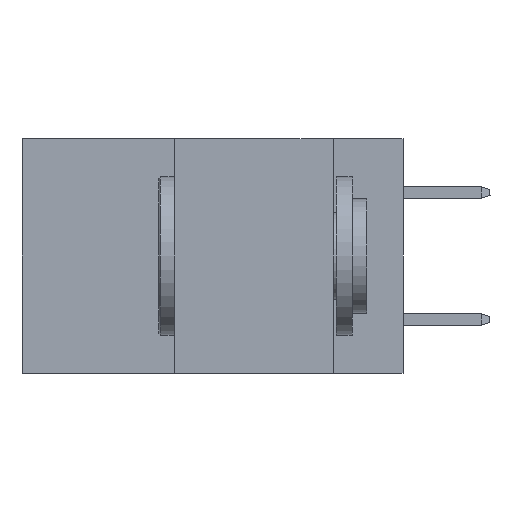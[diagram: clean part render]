
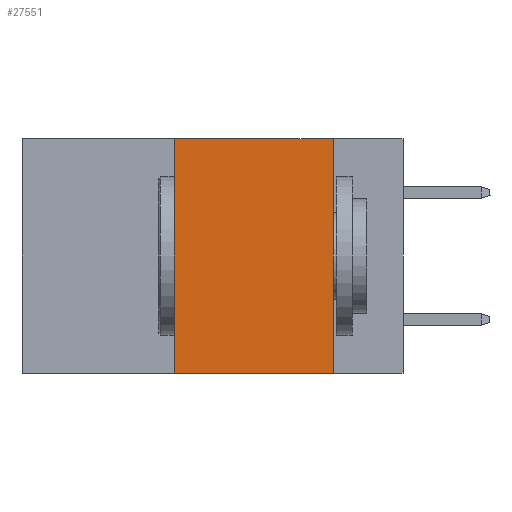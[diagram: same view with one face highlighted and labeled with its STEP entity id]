
A CAD part, left-side view. The second image highlights one B-rep face of the part: STEP entity #27551.
In plain terms, the highlighted planar face has unit normal (-1, 0, 0).
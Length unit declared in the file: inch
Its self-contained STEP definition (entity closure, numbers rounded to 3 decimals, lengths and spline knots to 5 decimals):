
#116 = AXIS2_PLACEMENT_3D ( 'NONE', #1748, #18415, #23609 ) ;
#1748 = CARTESIAN_POINT ( 'NONE',  ( 0., 0.6, 0. ) ) ;
#1804 = DIRECTION ( 'NONE',  ( 0., 0., -1. ) ) ;
#2273 = PLANE ( 'NONE',  #116 ) ;
#2361 = EDGE_CURVE ( 'NONE', #25182, #6002, #16049, .T. ) ;
#4284 = LINE ( 'NONE', #6936, #4635 ) ;
#4635 = VECTOR ( 'NONE', #1804, 39.37008 ) ;
#5375 = LINE ( 'NONE', #19546, #14119 ) ;
#6002 = VERTEX_POINT ( 'NONE', #31726 ) ;
#6936 = CARTESIAN_POINT ( 'NONE',  ( 0., 0.11, 0. ) ) ;
#7371 = CARTESIAN_POINT ( 'NONE',  ( 0., 0.36, 0. ) ) ;
#7825 = DIRECTION ( 'NONE',  ( 0., -1., 0. ) ) ;
#12424 = CARTESIAN_POINT ( 'NONE',  ( 0., 0.36, -0.37 ) ) ;
#14119 = VECTOR ( 'NONE', #18858, 39.37008 ) ;
#15386 = FACE_OUTER_BOUND ( 'NONE', #29943, .T. ) ;
#16049 = LINE ( 'NONE', #7371, #34654 ) ;
#16772 = VERTEX_POINT ( 'NONE', #32224 ) ;
#18169 = ORIENTED_EDGE ( 'NONE', *, *, #25236, .F. ) ;
#18415 = DIRECTION ( 'NONE',  ( 1., 0., 0. ) ) ;
#18463 = LINE ( 'NONE', #21332, #29448 ) ;
#18682 = ORIENTED_EDGE ( 'NONE', *, *, #2361, .F. ) ;
#18858 = DIRECTION ( 'NONE',  ( 0., -1., 0. ) ) ;
#19546 = CARTESIAN_POINT ( 'NONE',  ( 0., 0.6, -0.37 ) ) ;
#21332 = CARTESIAN_POINT ( 'NONE',  ( 0., 0.6, 0. ) ) ;
#23609 = DIRECTION ( 'NONE',  ( 0., 0., -1. ) ) ;
#25182 = VERTEX_POINT ( 'NONE', #12424 ) ;
#25222 = ORIENTED_EDGE ( 'NONE', *, *, #34970, .T. ) ;
#25236 = EDGE_CURVE ( 'NONE', #34313, #16772, #4284, .T. ) ;
#25976 = ORIENTED_EDGE ( 'NONE', *, *, #31154, .F. ) ;
#27551 = ADVANCED_FACE ( 'NONE', ( #15386 ), #2273, .F. ) ;
#29448 = VECTOR ( 'NONE', #7825, 39.37008 ) ;
#29943 = EDGE_LOOP ( 'NONE', ( #18169, #25976, #18682, #25222 ) ) ;
#31154 = EDGE_CURVE ( 'NONE', #6002, #34313, #18463, .T. ) ;
#31726 = CARTESIAN_POINT ( 'NONE',  ( 0., 0.36, 0. ) ) ;
#32224 = CARTESIAN_POINT ( 'NONE',  ( 0., 0.11, -0.37 ) ) ;
#33608 = DIRECTION ( 'NONE',  ( 0., 0., 1. ) ) ;
#33739 = CARTESIAN_POINT ( 'NONE',  ( 0., 0.11, 0. ) ) ;
#34313 = VERTEX_POINT ( 'NONE', #33739 ) ;
#34654 = VECTOR ( 'NONE', #33608, 39.37008 ) ;
#34970 = EDGE_CURVE ( 'NONE', #25182, #16772, #5375, .T. ) ;
